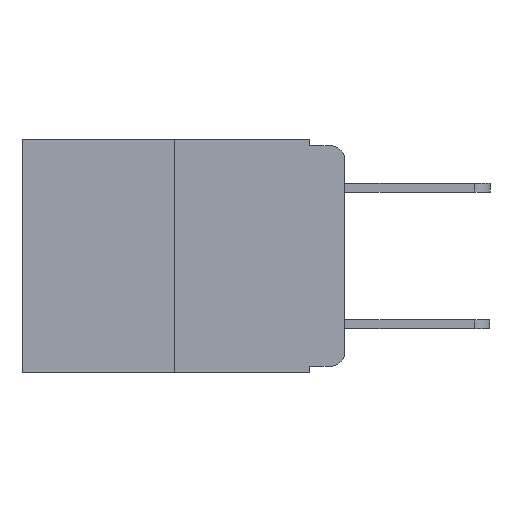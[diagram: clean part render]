
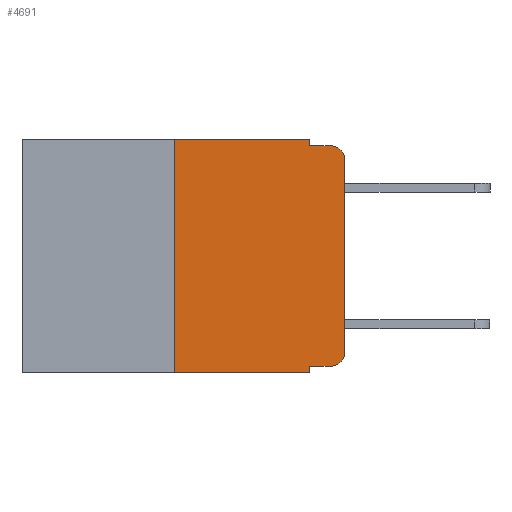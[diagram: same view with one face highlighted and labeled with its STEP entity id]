
A CAD part, left-side view. The second image highlights one B-rep face of the part: STEP entity #4691.
In plain terms, the highlighted planar face has unit normal (-1, 0, 0).
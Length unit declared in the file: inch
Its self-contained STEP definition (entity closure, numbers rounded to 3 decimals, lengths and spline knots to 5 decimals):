
#242 = VERTEX_POINT ( 'NONE', #1823 ) ;
#283 = ORIENTED_EDGE ( 'NONE', *, *, #4298, .T. ) ;
#453 = LINE ( 'NONE', #12778, #7901 ) ;
#916 = VERTEX_POINT ( 'NONE', #11136 ) ;
#976 = PLANE ( 'NONE',  #10145 ) ;
#1047 = CARTESIAN_POINT ( 'NONE',  ( 0., 0.051, 0. ) ) ;
#1823 = CARTESIAN_POINT ( 'NONE',  ( 0., 0.25, 0. ) ) ;
#2225 = VERTEX_POINT ( 'NONE', #7398 ) ;
#2229 = CARTESIAN_POINT ( 'NONE',  ( 0., 0.25, -0.343 ) ) ;
#2297 = DIRECTION ( 'NONE',  ( 0., -1., 0. ) ) ;
#2424 = LINE ( 'NONE', #4314, #9993 ) ;
#2979 = CIRCLE ( 'NONE', #7052, 0.02 ) ;
#3019 = VERTEX_POINT ( 'NONE', #9041 ) ;
#3034 = AXIS2_PLACEMENT_3D ( 'NONE', #6483, #12731, #7407 ) ;
#3128 = LINE ( 'NONE', #11701, #10791 ) ;
#3191 = EDGE_CURVE ( 'NONE', #242, #10624, #453, .T. ) ;
#3302 = DIRECTION ( 'NONE',  ( 0., 0., -1. ) ) ;
#3382 = ORIENTED_EDGE ( 'NONE', *, *, #9442, .T. ) ;
#3390 = ORIENTED_EDGE ( 'NONE', *, *, #11529, .F. ) ;
#3394 = CARTESIAN_POINT ( 'NONE',  ( 0., 0.02, -0.333 ) ) ;
#3601 = EDGE_CURVE ( 'NONE', #916, #2225, #4984, .T. ) ;
#3861 = VECTOR ( 'NONE', #11442, 39.37008 ) ;
#3903 = CARTESIAN_POINT ( 'NONE',  ( 0., 0.051, -0.01 ) ) ;
#3959 = VERTEX_POINT ( 'NONE', #2229 ) ;
#4220 = EDGE_CURVE ( 'NONE', #5418, #3019, #11407, .T. ) ;
#4298 = EDGE_CURVE ( 'NONE', #3019, #9073, #7916, .T. ) ;
#4314 = CARTESIAN_POINT ( 'NONE',  ( 0., 0.051, 0. ) ) ;
#4318 = CARTESIAN_POINT ( 'NONE',  ( 0., 0.473, 0. ) ) ;
#4513 = ORIENTED_EDGE ( 'NONE', *, *, #3601, .F. ) ;
#4691 = ADVANCED_FACE ( 'NONE', ( #8883 ), #976, .F. ) ;
#4742 = VECTOR ( 'NONE', #8477, 39.37008 ) ;
#4984 = LINE ( 'NONE', #1047, #12073 ) ;
#5026 = ORIENTED_EDGE ( 'NONE', *, *, #8393, .F. ) ;
#5126 = VERTEX_POINT ( 'NONE', #6190 ) ;
#5179 = ORIENTED_EDGE ( 'NONE', *, *, #4220, .T. ) ;
#5182 = ORIENTED_EDGE ( 'NONE', *, *, #11459, .T. ) ;
#5253 = VERTEX_POINT ( 'NONE', #3394 ) ;
#5363 = DIRECTION ( 'NONE',  ( 0., 0., -1. ) ) ;
#5401 = VECTOR ( 'NONE', #2297, 39.37008 ) ;
#5418 = VERTEX_POINT ( 'NONE', #12557 ) ;
#5643 = ORIENTED_EDGE ( 'NONE', *, *, #8251, .T. ) ;
#5981 = CARTESIAN_POINT ( 'NONE',  ( 0., 0.02, -0.313 ) ) ;
#6190 = CARTESIAN_POINT ( 'NONE',  ( 0., 0.051, -0.01 ) ) ;
#6459 = EDGE_LOOP ( 'NONE', ( #5179, #283, #5026, #12751, #10687, #3390, #3382, #4513, #5182, #5643 ) ) ;
#6483 = CARTESIAN_POINT ( 'NONE',  ( 0., 0.02, -0.03 ) ) ;
#7052 = AXIS2_PLACEMENT_3D ( 'NONE', #5981, #7225, #8558 ) ;
#7225 = DIRECTION ( 'NONE',  ( -1., 0., 0. ) ) ;
#7398 = CARTESIAN_POINT ( 'NONE',  ( 0., 0.051, -0.343 ) ) ;
#7407 = DIRECTION ( 'NONE',  ( 0., 0., -1. ) ) ;
#7587 = CARTESIAN_POINT ( 'NONE',  ( 0., 0.25, 0. ) ) ;
#7692 = LINE ( 'NONE', #7587, #4742 ) ;
#7901 = VECTOR ( 'NONE', #8237, 39.37008 ) ;
#7916 = CIRCLE ( 'NONE', #3034, 0.02 ) ;
#8237 = DIRECTION ( 'NONE',  ( 0., -1., 0. ) ) ;
#8251 = EDGE_CURVE ( 'NONE', #5253, #5418, #2979, .T. ) ;
#8393 = EDGE_CURVE ( 'NONE', #5126, #9073, #11386, .T. ) ;
#8477 = DIRECTION ( 'NONE',  ( 0., 0., 1. ) ) ;
#8558 = DIRECTION ( 'NONE',  ( 0., 0., -1. ) ) ;
#8678 = DIRECTION ( 'NONE',  ( 0., 0., -1. ) ) ;
#8883 = FACE_OUTER_BOUND ( 'NONE', #6459, .T. ) ;
#9041 = CARTESIAN_POINT ( 'NONE',  ( 0., 0., -0.03 ) ) ;
#9073 = VERTEX_POINT ( 'NONE', #9454 ) ;
#9180 = DIRECTION ( 'NONE',  ( 1., 0., 0. ) ) ;
#9291 = CARTESIAN_POINT ( 'NONE',  ( 0., 0.051, -0.333 ) ) ;
#9442 = EDGE_CURVE ( 'NONE', #3959, #2225, #3128, .T. ) ;
#9454 = CARTESIAN_POINT ( 'NONE',  ( 0., 0.02, -0.01 ) ) ;
#9528 = EDGE_CURVE ( 'NONE', #10624, #5126, #2424, .T. ) ;
#9920 = DIRECTION ( 'NONE',  ( 0., -1., 0. ) ) ;
#9946 = DIRECTION ( 'NONE',  ( 0., 0., 1. ) ) ;
#9993 = VECTOR ( 'NONE', #5363, 39.37008 ) ;
#10145 = AXIS2_PLACEMENT_3D ( 'NONE', #4318, #9180, #3302 ) ;
#10356 = LINE ( 'NONE', #9291, #5401 ) ;
#10624 = VERTEX_POINT ( 'NONE', #10829 ) ;
#10687 = ORIENTED_EDGE ( 'NONE', *, *, #3191, .F. ) ;
#10791 = VECTOR ( 'NONE', #9920, 39.37008 ) ;
#10829 = CARTESIAN_POINT ( 'NONE',  ( 0., 0.051, 0. ) ) ;
#11116 = VECTOR ( 'NONE', #9946, 39.37008 ) ;
#11136 = CARTESIAN_POINT ( 'NONE',  ( 0., 0.051, -0.333 ) ) ;
#11386 = LINE ( 'NONE', #3903, #3861 ) ;
#11407 = LINE ( 'NONE', #11720, #11116 ) ;
#11442 = DIRECTION ( 'NONE',  ( 0., -1., 0. ) ) ;
#11459 = EDGE_CURVE ( 'NONE', #916, #5253, #10356, .T. ) ;
#11529 = EDGE_CURVE ( 'NONE', #3959, #242, #7692, .T. ) ;
#11701 = CARTESIAN_POINT ( 'NONE',  ( 0., 0.473, -0.343 ) ) ;
#11720 = CARTESIAN_POINT ( 'NONE',  ( 0., 0., 0. ) ) ;
#12073 = VECTOR ( 'NONE', #8678, 39.37008 ) ;
#12557 = CARTESIAN_POINT ( 'NONE',  ( 0., 0., -0.313 ) ) ;
#12731 = DIRECTION ( 'NONE',  ( -1., 0., 0. ) ) ;
#12751 = ORIENTED_EDGE ( 'NONE', *, *, #9528, .F. ) ;
#12778 = CARTESIAN_POINT ( 'NONE',  ( 0., 0.473, 0. ) ) ;
